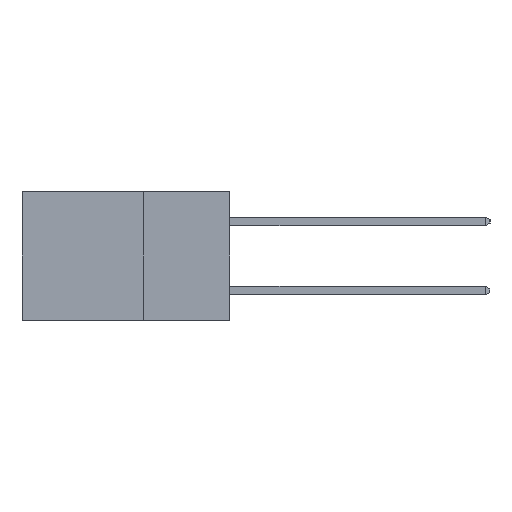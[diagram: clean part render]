
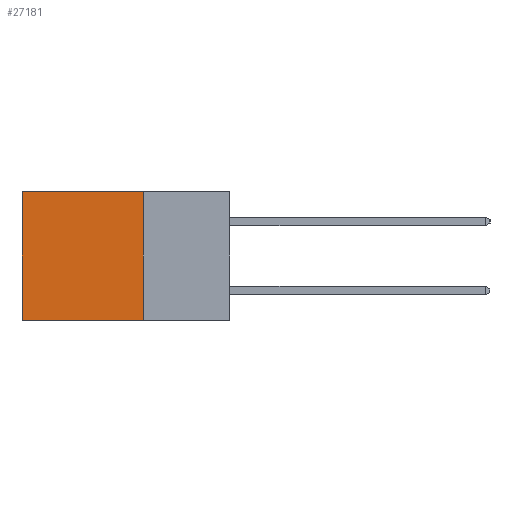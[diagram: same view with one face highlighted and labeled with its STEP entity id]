
A CAD part, left-side view. The second image highlights one B-rep face of the part: STEP entity #27181.
In plain terms, the highlighted planar face has unit normal (-1, 0, 0).
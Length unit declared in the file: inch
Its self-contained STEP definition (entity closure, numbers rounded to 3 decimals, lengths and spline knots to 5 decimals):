
#1672 = CARTESIAN_POINT ( 'NONE',  ( 0.298, 0.6, 0. ) ) ;
#1681 = VECTOR ( 'NONE', #24986, 39.37008 ) ;
#5501 = VERTEX_POINT ( 'NONE', #26401 ) ;
#6569 = ORIENTED_EDGE ( 'NONE', *, *, #16444, .T. ) ;
#6764 = VECTOR ( 'NONE', #11696, 39.37008 ) ;
#7618 = EDGE_LOOP ( 'NONE', ( #6569, #31973, #18088, #24895 ) ) ;
#8037 = VERTEX_POINT ( 'NONE', #16383 ) ;
#8597 = CARTESIAN_POINT ( 'NONE',  ( 0.298, 0.25, 0. ) ) ;
#8697 = CARTESIAN_POINT ( 'NONE',  ( 0.298, 0.25, 0. ) ) ;
#9181 = CARTESIAN_POINT ( 'NONE',  ( 0.298, 0.6, 0. ) ) ;
#9734 = VECTOR ( 'NONE', #10885, 39.37008 ) ;
#9887 = VECTOR ( 'NONE', #28550, 39.37008 ) ;
#10885 = DIRECTION ( 'NONE',  ( 0., 1., 0. ) ) ;
#11101 = PLANE ( 'NONE',  #28325 ) ;
#11696 = DIRECTION ( 'NONE',  ( 0., 0., -1. ) ) ;
#12559 = LINE ( 'NONE', #8697, #9887 ) ;
#13634 = DIRECTION ( 'NONE',  ( 0., 0., -1. ) ) ;
#15092 = LINE ( 'NONE', #22476, #1681 ) ;
#16383 = CARTESIAN_POINT ( 'NONE',  ( 0.298, 0.6, -0.37 ) ) ;
#16444 = EDGE_CURVE ( 'NONE', #26142, #8037, #26730, .T. ) ;
#17923 = VERTEX_POINT ( 'NONE', #29380 ) ;
#18088 = ORIENTED_EDGE ( 'NONE', *, *, #25284, .F. ) ;
#21560 = EDGE_CURVE ( 'NONE', #17923, #26142, #15092, .T. ) ;
#22326 = LINE ( 'NONE', #25921, #9734 ) ;
#22476 = CARTESIAN_POINT ( 'NONE',  ( 0.298, 0.25, 0. ) ) ;
#24895 = ORIENTED_EDGE ( 'NONE', *, *, #21560, .T. ) ;
#24986 = DIRECTION ( 'NONE',  ( 0., 1., 0. ) ) ;
#25284 = EDGE_CURVE ( 'NONE', #17923, #5501, #12559, .T. ) ;
#25921 = CARTESIAN_POINT ( 'NONE',  ( 0.298, 0.25, -0.37 ) ) ;
#26142 = VERTEX_POINT ( 'NONE', #1672 ) ;
#26401 = CARTESIAN_POINT ( 'NONE',  ( 0.298, 0.25, -0.37 ) ) ;
#26564 = FACE_OUTER_BOUND ( 'NONE', #7618, .T. ) ;
#26730 = LINE ( 'NONE', #9181, #6764 ) ;
#27105 = EDGE_CURVE ( 'NONE', #5501, #8037, #22326, .T. ) ;
#27181 = ADVANCED_FACE ( 'NONE', ( #26564 ), #11101, .F. ) ;
#28325 = AXIS2_PLACEMENT_3D ( 'NONE', #8597, #28557, #13634 ) ;
#28550 = DIRECTION ( 'NONE',  ( 0., 0., -1. ) ) ;
#28557 = DIRECTION ( 'NONE',  ( 1., 0., 0. ) ) ;
#29380 = CARTESIAN_POINT ( 'NONE',  ( 0.298, 0.25, 0. ) ) ;
#31973 = ORIENTED_EDGE ( 'NONE', *, *, #27105, .F. ) ;
